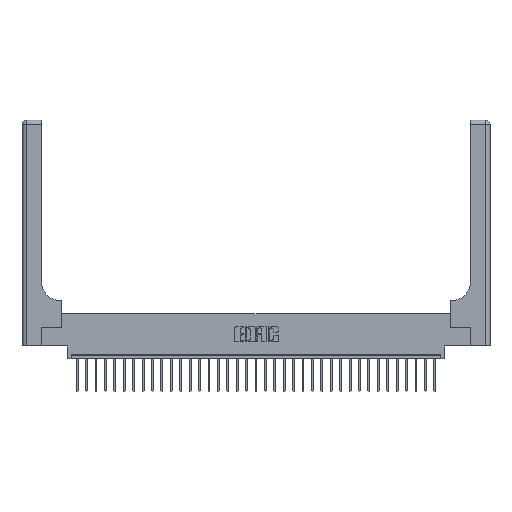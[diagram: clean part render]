
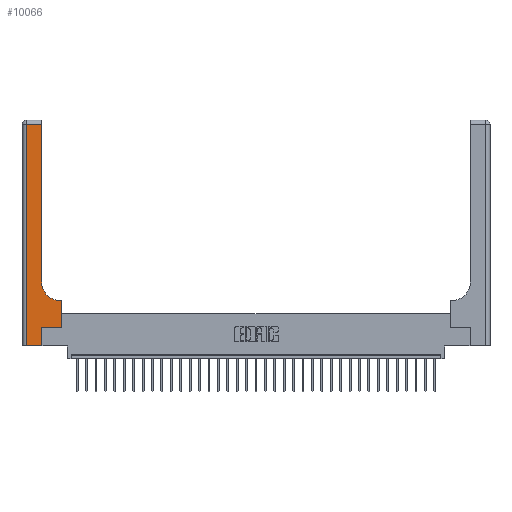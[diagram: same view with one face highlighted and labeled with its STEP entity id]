
A CAD part, top view. The second image highlights one B-rep face of the part: STEP entity #10066.
In plain terms, the highlighted planar face has unit normal (0, 0, 1).
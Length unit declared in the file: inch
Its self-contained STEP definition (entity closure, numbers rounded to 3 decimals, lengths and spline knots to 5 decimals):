
#482 = VERTEX_POINT ( 'NONE', #17774 ) ;
#910 = CARTESIAN_POINT ( 'NONE',  ( 0.06, 3., 0.37 ) ) ;
#1056 = CARTESIAN_POINT ( 'NONE',  ( 0., 3., 0.37 ) ) ;
#1371 = DIRECTION ( 'NONE',  ( 0., 1., 0. ) ) ;
#1480 = CARTESIAN_POINT ( 'NONE',  ( 0.265, 0., 0.37 ) ) ;
#1695 = EDGE_CURVE ( 'NONE', #14790, #29211, #23420, .T. ) ;
#1722 = LINE ( 'NONE', #10668, #22436 ) ;
#1766 = DIRECTION ( 'NONE',  ( 1., 0., 0. ) ) ;
#1804 = EDGE_CURVE ( 'NONE', #7019, #23750, #23727, .T. ) ;
#2100 = EDGE_CURVE ( 'NONE', #482, #16682, #1722, .T. ) ;
#2258 = CIRCLE ( 'NONE', #28279, 0.25 ) ;
#2449 = EDGE_CURVE ( 'NONE', #17876, #18928, #21350, .T. ) ;
#3128 = ORIENTED_EDGE ( 'NONE', *, *, #23766, .T. ) ;
#3445 = ORIENTED_EDGE ( 'NONE', *, *, #28527, .T. ) ;
#3470 = VECTOR ( 'NONE', #18246, 39.37008 ) ;
#4106 = CARTESIAN_POINT ( 'NONE',  ( 0.06, 0., 0.37 ) ) ;
#4584 = CARTESIAN_POINT ( 'NONE',  ( 0., 0., 0.37 ) ) ;
#5879 = VECTOR ( 'NONE', #9679, 39.37008 ) ;
#6095 = CARTESIAN_POINT ( 'NONE',  ( 0.51, 0.85, 0.37 ) ) ;
#6110 = CARTESIAN_POINT ( 'NONE',  ( 0.265, 0., 0.37 ) ) ;
#7019 = VERTEX_POINT ( 'NONE', #8105 ) ;
#7197 = DIRECTION ( 'NONE',  ( 1., 0., 0. ) ) ;
#7723 = CARTESIAN_POINT ( 'NONE',  ( 0.528, 0.25, 0.37 ) ) ;
#8105 = CARTESIAN_POINT ( 'NONE',  ( 0.26, 0.85, 0.37 ) ) ;
#8118 = FACE_OUTER_BOUND ( 'NONE', #14198, .T. ) ;
#8386 = VECTOR ( 'NONE', #1371, 39.37008 ) ;
#9611 = AXIS2_PLACEMENT_3D ( 'NONE', #1056, #15645, #10448 ) ;
#9679 = DIRECTION ( 'NONE',  ( -1., 0., 0. ) ) ;
#10066 = ADVANCED_FACE ( 'NONE', ( #8118 ), #24573, .F. ) ;
#10448 = DIRECTION ( 'NONE',  ( -1., 0., 0. ) ) ;
#10586 = VERTEX_POINT ( 'NONE', #18460 ) ;
#10668 = CARTESIAN_POINT ( 'NONE',  ( 0.265, 0.25, 0.37 ) ) ;
#10805 = EDGE_CURVE ( 'NONE', #10586, #17876, #17046, .T. ) ;
#12039 = ORIENTED_EDGE ( 'NONE', *, *, #1695, .T. ) ;
#13737 = CARTESIAN_POINT ( 'NONE',  ( 0.26, 0.6, 0.37 ) ) ;
#14198 = EDGE_LOOP ( 'NONE', ( #14328, #15664, #23438, #24388, #22280, #29914, #3445, #12039, #3128 ) ) ;
#14328 = ORIENTED_EDGE ( 'NONE', *, *, #1804, .T. ) ;
#14647 = EDGE_CURVE ( 'NONE', #18928, #482, #22709, .T. ) ;
#14790 = VERTEX_POINT ( 'NONE', #23442 ) ;
#14885 = LINE ( 'NONE', #26575, #5879 ) ;
#15645 = DIRECTION ( 'NONE',  ( 0., 0., -1. ) ) ;
#15664 = ORIENTED_EDGE ( 'NONE', *, *, #27271, .T. ) ;
#16677 = CARTESIAN_POINT ( 'NONE',  ( 0.51, 0.6, 0.37 ) ) ;
#16682 = VERTEX_POINT ( 'NONE', #7723 ) ;
#17046 = LINE ( 'NONE', #910, #23881 ) ;
#17418 = CARTESIAN_POINT ( 'NONE',  ( 0.26, 3., 0.37 ) ) ;
#17774 = CARTESIAN_POINT ( 'NONE',  ( 0.265, 0.25, 0.37 ) ) ;
#17876 = VERTEX_POINT ( 'NONE', #4106 ) ;
#18246 = DIRECTION ( 'NONE',  ( 0., 1., 0. ) ) ;
#18460 = CARTESIAN_POINT ( 'NONE',  ( 0.06, 2.94, 0.37 ) ) ;
#18928 = VERTEX_POINT ( 'NONE', #1480 ) ;
#20036 = DIRECTION ( 'NONE',  ( 1., 0., 0. ) ) ;
#21350 = LINE ( 'NONE', #4584, #23912 ) ;
#22142 = CARTESIAN_POINT ( 'NONE',  ( 0.528, 0.25, 0.37 ) ) ;
#22199 = DIRECTION ( 'NONE',  ( 0., 1., 0. ) ) ;
#22280 = ORIENTED_EDGE ( 'NONE', *, *, #14647, .T. ) ;
#22436 = VECTOR ( 'NONE', #20036, 39.37008 ) ;
#22709 = LINE ( 'NONE', #6110, #3470 ) ;
#22831 = CARTESIAN_POINT ( 'NONE',  ( 0.26, 2.94, 0.37 ) ) ;
#23126 = DIRECTION ( 'NONE',  ( -1., 0., 0. ) ) ;
#23420 = LINE ( 'NONE', #13737, #29724 ) ;
#23438 = ORIENTED_EDGE ( 'NONE', *, *, #10805, .T. ) ;
#23442 = CARTESIAN_POINT ( 'NONE',  ( 0.528, 0.6, 0.37 ) ) ;
#23727 = LINE ( 'NONE', #17418, #30214 ) ;
#23750 = VERTEX_POINT ( 'NONE', #22831 ) ;
#23766 = EDGE_CURVE ( 'NONE', #29211, #7019, #2258, .T. ) ;
#23881 = VECTOR ( 'NONE', #29026, 39.37008 ) ;
#23912 = VECTOR ( 'NONE', #7197, 39.37008 ) ;
#24388 = ORIENTED_EDGE ( 'NONE', *, *, #2449, .T. ) ;
#24573 = PLANE ( 'NONE',  #9611 ) ;
#24995 = DIRECTION ( 'NONE',  ( 0., 0., -1. ) ) ;
#26575 = CARTESIAN_POINT ( 'NONE',  ( 0., 2.94, 0.37 ) ) ;
#27271 = EDGE_CURVE ( 'NONE', #23750, #10586, #14885, .T. ) ;
#28279 = AXIS2_PLACEMENT_3D ( 'NONE', #6095, #24995, #1766 ) ;
#28527 = EDGE_CURVE ( 'NONE', #16682, #14790, #29765, .T. ) ;
#29026 = DIRECTION ( 'NONE',  ( 0., -1., 0. ) ) ;
#29211 = VERTEX_POINT ( 'NONE', #16677 ) ;
#29724 = VECTOR ( 'NONE', #23126, 39.37008 ) ;
#29765 = LINE ( 'NONE', #22142, #8386 ) ;
#29914 = ORIENTED_EDGE ( 'NONE', *, *, #2100, .T. ) ;
#30214 = VECTOR ( 'NONE', #22199, 39.37008 ) ;
